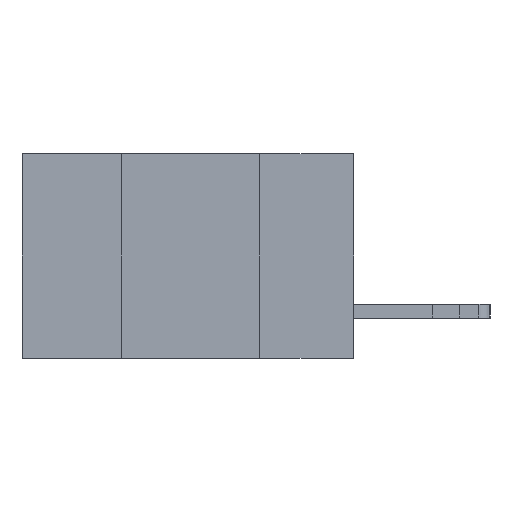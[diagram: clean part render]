
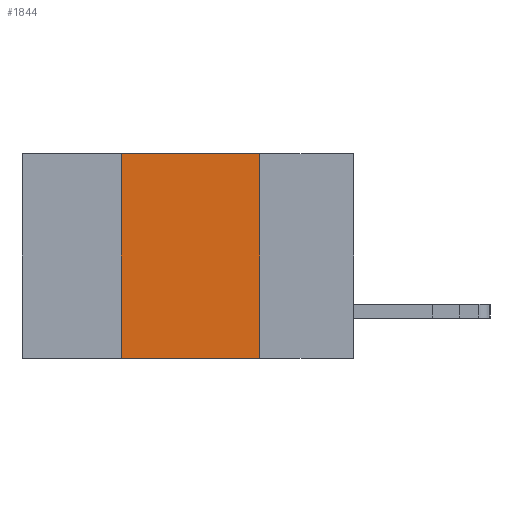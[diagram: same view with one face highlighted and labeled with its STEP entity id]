
A CAD part, left-side view. The second image highlights one B-rep face of the part: STEP entity #1844.
In plain terms, the highlighted planar face has unit normal (-1, 0, 0).
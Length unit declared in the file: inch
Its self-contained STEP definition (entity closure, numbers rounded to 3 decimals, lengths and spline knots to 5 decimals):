
#22 = ORIENTED_EDGE ( 'NONE', *, *, #8303, .F. ) ;
#474 = DIRECTION ( 'NONE',  ( 0., -1., 0. ) ) ;
#606 = ORIENTED_EDGE ( 'NONE', *, *, #1684, .F. ) ;
#635 = CARTESIAN_POINT ( 'NONE',  ( 0., 0.6, -0.37 ) ) ;
#956 = VERTEX_POINT ( 'NONE', #2132 ) ;
#1559 = VERTEX_POINT ( 'NONE', #15324 ) ;
#1605 = LINE ( 'NONE', #635, #3055 ) ;
#1684 = EDGE_CURVE ( 'NONE', #10272, #11750, #8619, .T. ) ;
#1844 = ADVANCED_FACE ( 'NONE', ( #2521 ), #7631, .F. ) ;
#2132 = CARTESIAN_POINT ( 'NONE',  ( 0., 0.17, -0.37 ) ) ;
#2521 = FACE_OUTER_BOUND ( 'NONE', #8394, .T. ) ;
#3055 = VECTOR ( 'NONE', #6710, 39.37008 ) ;
#3160 = LINE ( 'NONE', #12912, #3602 ) ;
#3602 = VECTOR ( 'NONE', #15699, 39.37008 ) ;
#3705 = EDGE_CURVE ( 'NONE', #10272, #956, #1605, .T. ) ;
#5244 = CARTESIAN_POINT ( 'NONE',  ( 0., 0.6, 0. ) ) ;
#5874 = VECTOR ( 'NONE', #15907, 39.37008 ) ;
#6206 = VECTOR ( 'NONE', #474, 39.37008 ) ;
#6322 = DIRECTION ( 'NONE',  ( 0., 0., -1. ) ) ;
#6626 = EDGE_CURVE ( 'NONE', #1559, #956, #3160, .T. ) ;
#6710 = DIRECTION ( 'NONE',  ( 0., -1., 0. ) ) ;
#7167 = CARTESIAN_POINT ( 'NONE',  ( 0., 0.42, 0. ) ) ;
#7380 = ORIENTED_EDGE ( 'NONE', *, *, #6626, .F. ) ;
#7631 = PLANE ( 'NONE',  #15009 ) ;
#8303 = EDGE_CURVE ( 'NONE', #11750, #1559, #9146, .T. ) ;
#8394 = EDGE_LOOP ( 'NONE', ( #7380, #22, #606, #8651 ) ) ;
#8619 = LINE ( 'NONE', #7167, #5874 ) ;
#8651 = ORIENTED_EDGE ( 'NONE', *, *, #3705, .T. ) ;
#8696 = DIRECTION ( 'NONE',  ( 1., 0., 0. ) ) ;
#8997 = CARTESIAN_POINT ( 'NONE',  ( 0., 0.6, 0. ) ) ;
#9146 = LINE ( 'NONE', #5244, #6206 ) ;
#10272 = VERTEX_POINT ( 'NONE', #12565 ) ;
#11750 = VERTEX_POINT ( 'NONE', #15531 ) ;
#12565 = CARTESIAN_POINT ( 'NONE',  ( 0., 0.42, -0.37 ) ) ;
#12912 = CARTESIAN_POINT ( 'NONE',  ( 0., 0.17, 0. ) ) ;
#15009 = AXIS2_PLACEMENT_3D ( 'NONE', #8997, #8696, #6322 ) ;
#15324 = CARTESIAN_POINT ( 'NONE',  ( 0., 0.17, 0. ) ) ;
#15531 = CARTESIAN_POINT ( 'NONE',  ( 0., 0.42, 0. ) ) ;
#15699 = DIRECTION ( 'NONE',  ( 0., 0., -1. ) ) ;
#15907 = DIRECTION ( 'NONE',  ( 0., 0., 1. ) ) ;
